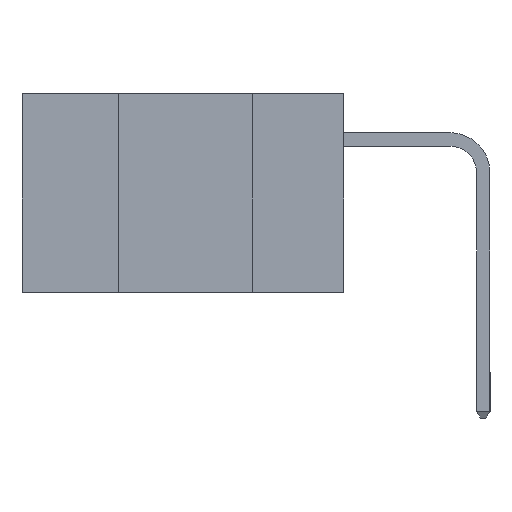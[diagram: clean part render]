
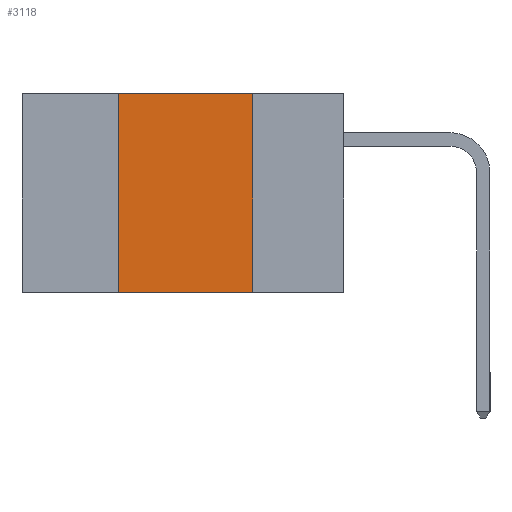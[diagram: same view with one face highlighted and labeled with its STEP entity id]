
A CAD part, left-side view. The second image highlights one B-rep face of the part: STEP entity #3118.
In plain terms, the highlighted planar face has unit normal (-1, 0, 0).
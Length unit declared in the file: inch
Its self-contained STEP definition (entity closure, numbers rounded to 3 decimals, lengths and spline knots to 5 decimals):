
#143 = DIRECTION ( 'NONE',  ( 0., 0., -1. ) ) ;
#619 = VECTOR ( 'NONE', #1521, 39.37008 ) ;
#773 = EDGE_CURVE ( 'NONE', #6634, #2533, #4265, .T. ) ;
#888 = ORIENTED_EDGE ( 'NONE', *, *, #6493, .T. ) ;
#1120 = CARTESIAN_POINT ( 'NONE',  ( 0., 0.17, 0. ) ) ;
#1134 = CARTESIAN_POINT ( 'NONE',  ( 0., 0.6, 0. ) ) ;
#1380 = CARTESIAN_POINT ( 'NONE',  ( 0., 0.6, 0. ) ) ;
#1521 = DIRECTION ( 'NONE',  ( 0., 0., 1. ) ) ;
#2482 = ORIENTED_EDGE ( 'NONE', *, *, #8027, .F. ) ;
#2533 = VERTEX_POINT ( 'NONE', #4076 ) ;
#3118 = ADVANCED_FACE ( 'NONE', ( #9699 ), #8047, .F. ) ;
#3498 = ORIENTED_EDGE ( 'NONE', *, *, #773, .F. ) ;
#4032 = LINE ( 'NONE', #5652, #8358 ) ;
#4076 = CARTESIAN_POINT ( 'NONE',  ( 0., 0.17, -0.37 ) ) ;
#4256 = VERTEX_POINT ( 'NONE', #10316 ) ;
#4265 = LINE ( 'NONE', #6756, #8592 ) ;
#5581 = DIRECTION ( 'NONE',  ( 1., 0., 0. ) ) ;
#5652 = CARTESIAN_POINT ( 'NONE',  ( 0., 0.6, -0.37 ) ) ;
#6430 = LINE ( 'NONE', #9738, #619 ) ;
#6447 = DIRECTION ( 'NONE',  ( 0., 0., -1. ) ) ;
#6493 = EDGE_CURVE ( 'NONE', #4256, #2533, #4032, .T. ) ;
#6634 = VERTEX_POINT ( 'NONE', #1120 ) ;
#6756 = CARTESIAN_POINT ( 'NONE',  ( 0., 0.17, -0.37 ) ) ;
#7022 = CARTESIAN_POINT ( 'NONE',  ( 0., 0.42, 0. ) ) ;
#7089 = ORIENTED_EDGE ( 'NONE', *, *, #7613, .F. ) ;
#7531 = LINE ( 'NONE', #1134, #9371 ) ;
#7613 = EDGE_CURVE ( 'NONE', #7989, #6634, #7531, .T. ) ;
#7989 = VERTEX_POINT ( 'NONE', #7022 ) ;
#8027 = EDGE_CURVE ( 'NONE', #4256, #7989, #6430, .T. ) ;
#8047 = PLANE ( 'NONE',  #10017 ) ;
#8358 = VECTOR ( 'NONE', #8952, 39.37008 ) ;
#8592 = VECTOR ( 'NONE', #143, 39.37008 ) ;
#8952 = DIRECTION ( 'NONE',  ( 0., -1., 0. ) ) ;
#9371 = VECTOR ( 'NONE', #10244, 39.37008 ) ;
#9699 = FACE_OUTER_BOUND ( 'NONE', #10097, .T. ) ;
#9738 = CARTESIAN_POINT ( 'NONE',  ( 0., 0.42, -0.37 ) ) ;
#10017 = AXIS2_PLACEMENT_3D ( 'NONE', #1380, #5581, #6447 ) ;
#10097 = EDGE_LOOP ( 'NONE', ( #3498, #7089, #2482, #888 ) ) ;
#10244 = DIRECTION ( 'NONE',  ( 0., -1., 0. ) ) ;
#10316 = CARTESIAN_POINT ( 'NONE',  ( 0., 0.42, -0.37 ) ) ;
